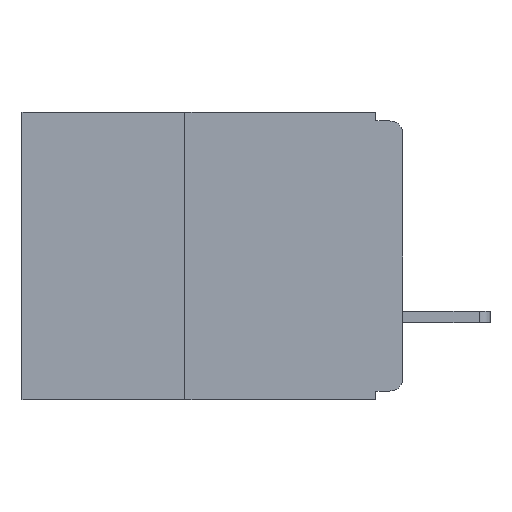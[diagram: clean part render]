
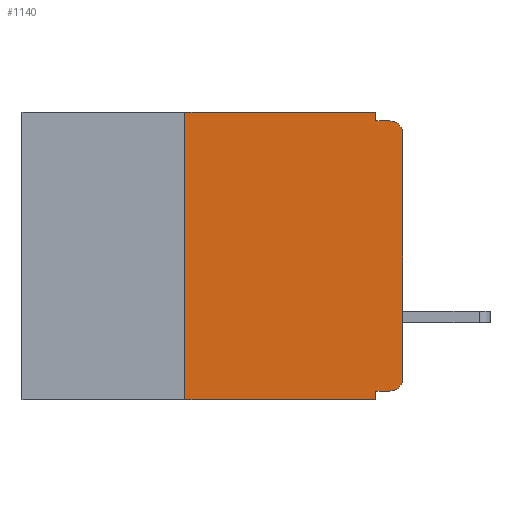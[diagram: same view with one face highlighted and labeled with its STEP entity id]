
A CAD part, left-side view. The second image highlights one B-rep face of the part: STEP entity #1140.
In plain terms, the highlighted planar face has unit normal (-1, 0, 0).
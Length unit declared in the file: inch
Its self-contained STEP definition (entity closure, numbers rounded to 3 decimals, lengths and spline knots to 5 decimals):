
#216 = CARTESIAN_POINT ( 'NONE',  ( 0., 0.437, 0. ) ) ;
#394 = EDGE_CURVE ( 'NONE', #5376, #3980, #7274, .T. ) ;
#633 = ORIENTED_EDGE ( 'NONE', *, *, #1557, .F. ) ;
#814 = VERTEX_POINT ( 'NONE', #12682 ) ;
#820 = DIRECTION ( 'NONE',  ( 0., 0., -1. ) ) ;
#833 = DIRECTION ( 'NONE',  ( 0., -1., 0. ) ) ;
#963 = AXIS2_PLACEMENT_3D ( 'NONE', #12897, #12834, #12656 ) ;
#1073 = DIRECTION ( 'NONE',  ( -1., 0., 0. ) ) ;
#1140 = ADVANCED_FACE ( 'NONE', ( #14259 ), #1817, .F. ) ;
#1216 = EDGE_CURVE ( 'NONE', #5411, #11727, #6256, .T. ) ;
#1225 = EDGE_CURVE ( 'NONE', #10522, #14112, #12781, .T. ) ;
#1307 = CARTESIAN_POINT ( 'NONE',  ( 0., 0.015, -0.025 ) ) ;
#1413 = EDGE_CURVE ( 'NONE', #12972, #3980, #11048, .T. ) ;
#1445 = CIRCLE ( 'NONE', #963, 0.015 ) ;
#1455 = CARTESIAN_POINT ( 'NONE',  ( 0., 0.015, -0.32 ) ) ;
#1557 = EDGE_CURVE ( 'NONE', #11727, #5376, #6241, .T. ) ;
#1578 = CARTESIAN_POINT ( 'NONE',  ( 0., 0.437, -0.33 ) ) ;
#1807 = EDGE_CURVE ( 'NONE', #9556, #5411, #14405, .T. ) ;
#1817 = PLANE ( 'NONE',  #4142 ) ;
#2097 = EDGE_CURVE ( 'NONE', #10522, #814, #1445, .T. ) ;
#2225 = EDGE_CURVE ( 'NONE', #9556, #14491, #14568, .T. ) ;
#2376 = CARTESIAN_POINT ( 'NONE',  ( 0., 0.25, -0.33 ) ) ;
#2774 = VECTOR ( 'NONE', #6544, 39.37008 ) ;
#2800 = EDGE_CURVE ( 'NONE', #14112, #14491, #12128, .T. ) ;
#3419 = CARTESIAN_POINT ( 'NONE',  ( 0., 0., 0. ) ) ;
#3537 = DIRECTION ( 'NONE',  ( 0., -1., 0. ) ) ;
#3890 = VECTOR ( 'NONE', #3537, 39.37008 ) ;
#3980 = VERTEX_POINT ( 'NONE', #10269 ) ;
#4142 = AXIS2_PLACEMENT_3D ( 'NONE', #216, #14385, #14103 ) ;
#4252 = CARTESIAN_POINT ( 'NONE',  ( 0., 0., -0.01 ) ) ;
#4638 = ORIENTED_EDGE ( 'NONE', *, *, #1216, .F. ) ;
#4737 = CARTESIAN_POINT ( 'NONE',  ( 0., 0.25, -0.33 ) ) ;
#4818 = DIRECTION ( 'NONE',  ( 0., 0., 1. ) ) ;
#5376 = VERTEX_POINT ( 'NONE', #11942 ) ;
#5411 = VERTEX_POINT ( 'NONE', #11154 ) ;
#5661 = DIRECTION ( 'NONE',  ( 0., 1., 0. ) ) ;
#5945 = CARTESIAN_POINT ( 'NONE',  ( 0., 0., -0.32 ) ) ;
#6241 = LINE ( 'NONE', #10307, #14788 ) ;
#6256 = LINE ( 'NONE', #9817, #2774 ) ;
#6444 = ORIENTED_EDGE ( 'NONE', *, *, #1413, .T. ) ;
#6544 = DIRECTION ( 'NONE',  ( 0., -1., 0. ) ) ;
#6681 = CARTESIAN_POINT ( 'NONE',  ( 0., 0., -0.025 ) ) ;
#6820 = ORIENTED_EDGE ( 'NONE', *, *, #394, .F. ) ;
#6833 = ORIENTED_EDGE ( 'NONE', *, *, #2097, .T. ) ;
#6981 = CARTESIAN_POINT ( 'NONE',  ( 0., 0.031, 0. ) ) ;
#7230 = AXIS2_PLACEMENT_3D ( 'NONE', #1307, #1073, #820 ) ;
#7274 = LINE ( 'NONE', #4252, #3890 ) ;
#7508 = VECTOR ( 'NONE', #12165, 39.37008 ) ;
#7806 = CARTESIAN_POINT ( 'NONE',  ( 0., 0.031, -0.33 ) ) ;
#7825 = ORIENTED_EDGE ( 'NONE', *, *, #2225, .T. ) ;
#8092 = EDGE_CURVE ( 'NONE', #814, #12972, #15943, .T. ) ;
#9176 = VECTOR ( 'NONE', #5661, 39.37008 ) ;
#9556 = VERTEX_POINT ( 'NONE', #2376 ) ;
#9817 = CARTESIAN_POINT ( 'NONE',  ( 0., 0.437, 0. ) ) ;
#10269 = CARTESIAN_POINT ( 'NONE',  ( 0., 0.015, -0.01 ) ) ;
#10307 = CARTESIAN_POINT ( 'NONE',  ( 0., 0.031, 0. ) ) ;
#10522 = VERTEX_POINT ( 'NONE', #1455 ) ;
#10945 = CARTESIAN_POINT ( 'NONE',  ( 0., 0.031, -0.32 ) ) ;
#11048 = CIRCLE ( 'NONE', #7230, 0.015 ) ;
#11154 = CARTESIAN_POINT ( 'NONE',  ( 0., 0.25, 0. ) ) ;
#11320 = DIRECTION ( 'NONE',  ( 0., 0., -1. ) ) ;
#11405 = VECTOR ( 'NONE', #833, 39.37008 ) ;
#11727 = VERTEX_POINT ( 'NONE', #6981 ) ;
#11836 = ORIENTED_EDGE ( 'NONE', *, *, #1225, .F. ) ;
#11942 = CARTESIAN_POINT ( 'NONE',  ( 0., 0.031, -0.01 ) ) ;
#12128 = LINE ( 'NONE', #12345, #14908 ) ;
#12165 = DIRECTION ( 'NONE',  ( 0., 0., 1. ) ) ;
#12306 = DIRECTION ( 'NONE',  ( 0., 0., -1. ) ) ;
#12345 = CARTESIAN_POINT ( 'NONE',  ( 0., 0.031, -0.33 ) ) ;
#12656 = DIRECTION ( 'NONE',  ( 0., 0., -1. ) ) ;
#12682 = CARTESIAN_POINT ( 'NONE',  ( 0., 0., -0.305 ) ) ;
#12769 = ORIENTED_EDGE ( 'NONE', *, *, #1807, .F. ) ;
#12781 = LINE ( 'NONE', #5945, #9176 ) ;
#12834 = DIRECTION ( 'NONE',  ( -1., 0., 0. ) ) ;
#12897 = CARTESIAN_POINT ( 'NONE',  ( 0., 0.015, -0.305 ) ) ;
#12972 = VERTEX_POINT ( 'NONE', #6681 ) ;
#14036 = VECTOR ( 'NONE', #4818, 39.37008 ) ;
#14103 = DIRECTION ( 'NONE',  ( 0., 0., -1. ) ) ;
#14112 = VERTEX_POINT ( 'NONE', #10945 ) ;
#14259 = FACE_OUTER_BOUND ( 'NONE', #14750, .T. ) ;
#14385 = DIRECTION ( 'NONE',  ( 1., 0., 0. ) ) ;
#14405 = LINE ( 'NONE', #4737, #14036 ) ;
#14491 = VERTEX_POINT ( 'NONE', #7806 ) ;
#14568 = LINE ( 'NONE', #1578, #11405 ) ;
#14614 = ORIENTED_EDGE ( 'NONE', *, *, #2800, .F. ) ;
#14750 = EDGE_LOOP ( 'NONE', ( #15684, #6444, #6820, #633, #4638, #12769, #7825, #14614, #11836, #6833 ) ) ;
#14788 = VECTOR ( 'NONE', #11320, 39.37008 ) ;
#14908 = VECTOR ( 'NONE', #12306, 39.37008 ) ;
#15684 = ORIENTED_EDGE ( 'NONE', *, *, #8092, .T. ) ;
#15943 = LINE ( 'NONE', #3419, #7508 ) ;
